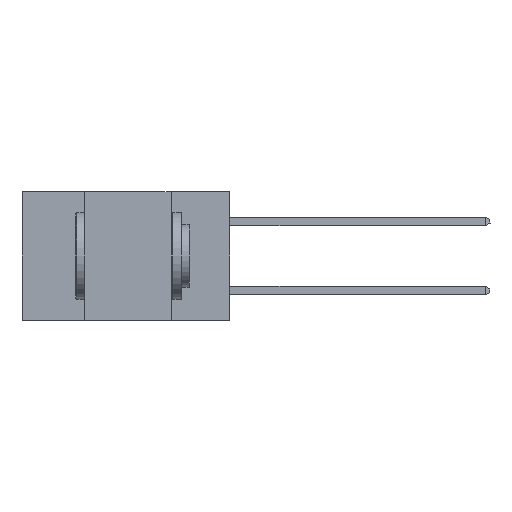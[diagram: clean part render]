
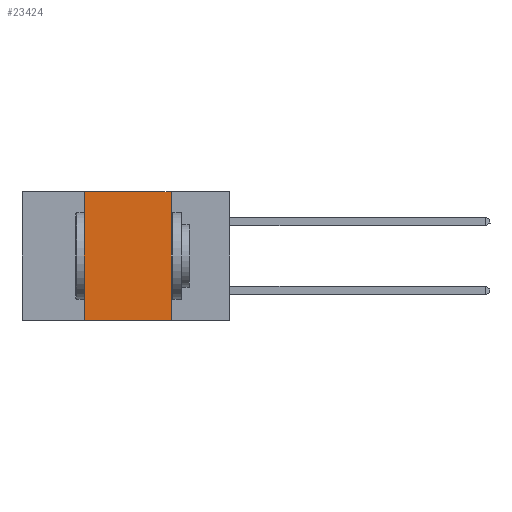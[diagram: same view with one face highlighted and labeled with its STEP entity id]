
A CAD part, left-side view. The second image highlights one B-rep face of the part: STEP entity #23424.
In plain terms, the highlighted planar face has unit normal (-1, 0, 0).
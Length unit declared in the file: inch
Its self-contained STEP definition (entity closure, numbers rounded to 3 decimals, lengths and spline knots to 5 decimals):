
#488 = EDGE_CURVE ( 'NONE', #12462, #19204, #20398, .T. ) ;
#4485 = ORIENTED_EDGE ( 'NONE', *, *, #488, .F. ) ;
#5229 = CARTESIAN_POINT ( 'NONE',  ( 0., 0.42, 0. ) ) ;
#8865 = ORIENTED_EDGE ( 'NONE', *, *, #30436, .F. ) ;
#9248 = DIRECTION ( 'NONE',  ( 1., 0., 0. ) ) ;
#9277 = LINE ( 'NONE', #5229, #16227 ) ;
#12435 = VECTOR ( 'NONE', #13288, 39.37008 ) ;
#12462 = VERTEX_POINT ( 'NONE', #29852 ) ;
#12785 = EDGE_CURVE ( 'NONE', #26704, #19204, #26850, .T. ) ;
#13288 = DIRECTION ( 'NONE',  ( 0., -1., 0. ) ) ;
#13341 = ORIENTED_EDGE ( 'NONE', *, *, #16293, .F. ) ;
#15050 = CARTESIAN_POINT ( 'NONE',  ( 0., 0.42, 0. ) ) ;
#15649 = ORIENTED_EDGE ( 'NONE', *, *, #12785, .T. ) ;
#16227 = VECTOR ( 'NONE', #18211, 39.37008 ) ;
#16293 = EDGE_CURVE ( 'NONE', #29729, #12462, #19099, .T. ) ;
#18211 = DIRECTION ( 'NONE',  ( 0., 0., 1. ) ) ;
#18311 = VECTOR ( 'NONE', #29152, 39.37008 ) ;
#18513 = CARTESIAN_POINT ( 'NONE',  ( 0., 0.6, -0.37 ) ) ;
#19099 = LINE ( 'NONE', #26674, #18311 ) ;
#19204 = VERTEX_POINT ( 'NONE', #27919 ) ;
#19566 = CARTESIAN_POINT ( 'NONE',  ( 0., 0.6, 0. ) ) ;
#20398 = LINE ( 'NONE', #29929, #32557 ) ;
#21666 = CARTESIAN_POINT ( 'NONE',  ( 0., 0.42, -0.37 ) ) ;
#22515 = AXIS2_PLACEMENT_3D ( 'NONE', #19566, #9248, #27197 ) ;
#22924 = FACE_OUTER_BOUND ( 'NONE', #25810, .T. ) ;
#23424 = ADVANCED_FACE ( 'NONE', ( #22924 ), #24669, .F. ) ;
#24669 = PLANE ( 'NONE',  #22515 ) ;
#25810 = EDGE_LOOP ( 'NONE', ( #4485, #13341, #8865, #15649 ) ) ;
#26674 = CARTESIAN_POINT ( 'NONE',  ( 0., 0.6, 0. ) ) ;
#26704 = VERTEX_POINT ( 'NONE', #21666 ) ;
#26850 = LINE ( 'NONE', #18513, #12435 ) ;
#27197 = DIRECTION ( 'NONE',  ( 0., 0., -1. ) ) ;
#27919 = CARTESIAN_POINT ( 'NONE',  ( 0., 0.17, -0.37 ) ) ;
#29152 = DIRECTION ( 'NONE',  ( 0., -1., 0. ) ) ;
#29729 = VERTEX_POINT ( 'NONE', #15050 ) ;
#29852 = CARTESIAN_POINT ( 'NONE',  ( 0., 0.17, 0. ) ) ;
#29929 = CARTESIAN_POINT ( 'NONE',  ( 0., 0.17, 0. ) ) ;
#30031 = DIRECTION ( 'NONE',  ( 0., 0., -1. ) ) ;
#30436 = EDGE_CURVE ( 'NONE', #26704, #29729, #9277, .T. ) ;
#32557 = VECTOR ( 'NONE', #30031, 39.37008 ) ;
